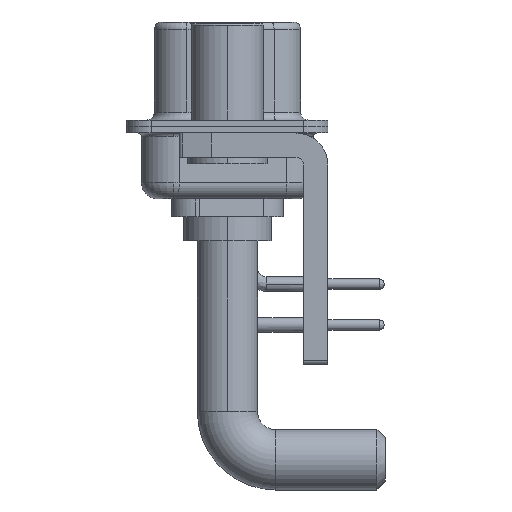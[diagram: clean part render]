
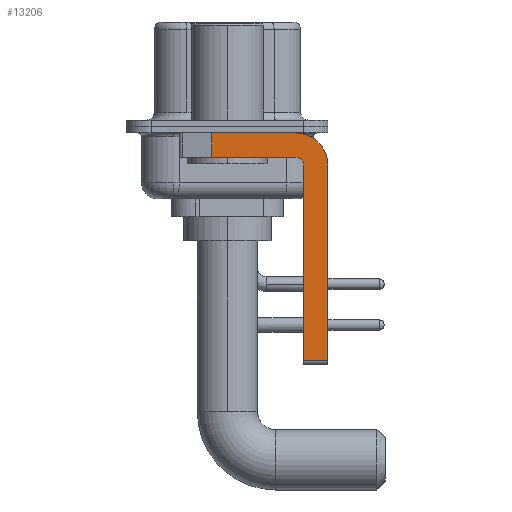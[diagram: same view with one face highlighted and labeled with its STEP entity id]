
A CAD part, left-side view. The second image highlights one B-rep face of the part: STEP entity #13206.
In plain terms, the highlighted planar face has unit normal (-1, 0, 0).
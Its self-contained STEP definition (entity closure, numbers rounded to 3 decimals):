
#13 = ORIENTED_EDGE ( 'NONE', *, *, #18868, .T. ) ;
#313 = ORIENTED_EDGE ( 'NONE', *, *, #8217, .F. ) ;
#1547 = LINE ( 'NONE', #5778, #13247 ) ;
#1688 = VERTEX_POINT ( 'NONE', #19954 ) ;
#1714 = CARTESIAN_POINT ( 'NONE',  ( -2.9, -4.25, -2.4 ) ) ;
#1807 = AXIS2_PLACEMENT_3D ( 'NONE', #6169, #8895, #23213 ) ;
#2792 = EDGE_CURVE ( 'NONE', #22148, #3441, #10200, .T. ) ;
#3090 = ORIENTED_EDGE ( 'NONE', *, *, #12988, .T. ) ;
#3268 = CARTESIAN_POINT ( 'NONE',  ( -2.9, 0.978, -0.4 ) ) ;
#3317 = DIRECTION ( 'NONE',  ( 0., -1., 0. ) ) ;
#3441 = VERTEX_POINT ( 'NONE', #26065 ) ;
#3748 = CARTESIAN_POINT ( 'NONE',  ( -2.9, -4.25, -1.9 ) ) ;
#3822 = CARTESIAN_POINT ( 'NONE',  ( -2.9, -4.25, -1.9 ) ) ;
#3893 = CARTESIAN_POINT ( 'NONE',  ( -2.9, -4.25, -0.4 ) ) ;
#4462 = VERTEX_POINT ( 'NONE', #10042 ) ;
#5024 = AXIS2_PLACEMENT_3D ( 'NONE', #24545, #5852, #7634 ) ;
#5320 = VECTOR ( 'NONE', #10472, 1000. ) ;
#5778 = CARTESIAN_POINT ( 'NONE',  ( -2.9, -4.25, -14.55 ) ) ;
#5852 = DIRECTION ( 'NONE',  ( -1., 0., 0. ) ) ;
#6034 = CARTESIAN_POINT ( 'NONE',  ( -2.9, -6.25, -2.4 ) ) ;
#6169 = CARTESIAN_POINT ( 'NONE',  ( -2.9, -4.25, -2.4 ) ) ;
#6187 = DIRECTION ( 'NONE',  ( 0., 0., -1. ) ) ;
#6374 = VECTOR ( 'NONE', #11959, 1000. ) ;
#6579 = LINE ( 'NONE', #23232, #15756 ) ;
#6833 = EDGE_CURVE ( 'NONE', #8709, #26379, #17943, .T. ) ;
#7211 = VECTOR ( 'NONE', #3317, 1000. ) ;
#7634 = DIRECTION ( 'NONE',  ( 0., 0., 1. ) ) ;
#8217 = EDGE_CURVE ( 'NONE', #25365, #16747, #22420, .T. ) ;
#8627 = PLANE ( 'NONE',  #1807 ) ;
#8709 = VERTEX_POINT ( 'NONE', #3822 ) ;
#8895 = DIRECTION ( 'NONE',  ( 1., 0., 0. ) ) ;
#10042 = CARTESIAN_POINT ( 'NONE',  ( -2.9, -4.75, -2.4 ) ) ;
#10200 = LINE ( 'NONE', #26837, #5320 ) ;
#10472 = DIRECTION ( 'NONE',  ( 0., 0., -1. ) ) ;
#11743 = LINE ( 'NONE', #18270, #22120 ) ;
#11871 = DIRECTION ( 'NONE',  ( 0., 0., 1. ) ) ;
#11959 = DIRECTION ( 'NONE',  ( 0., 1., 0. ) ) ;
#12988 = EDGE_CURVE ( 'NONE', #25365, #26379, #6579, .T. ) ;
#13206 = ADVANCED_FACE ( 'NONE', ( #25126 ), #8627, .F. ) ;
#13247 = VECTOR ( 'NONE', #22174, 1000. ) ;
#13322 = EDGE_LOOP ( 'NONE', ( #313, #3090, #19297, #14415, #20911, #13, #19116, #15576 ) ) ;
#13759 = CIRCLE ( 'NONE', #5024, 0.5 ) ;
#14134 = DIRECTION ( 'NONE',  ( 1., 0., 0. ) ) ;
#14415 = ORIENTED_EDGE ( 'NONE', *, *, #20709, .F. ) ;
#15576 = ORIENTED_EDGE ( 'NONE', *, *, #18301, .F. ) ;
#15756 = VECTOR ( 'NONE', #6187, 1000. ) ;
#16747 = VERTEX_POINT ( 'NONE', #3893 ) ;
#17943 = LINE ( 'NONE', #3748, #6374 ) ;
#18270 = CARTESIAN_POINT ( 'NONE',  ( -2.9, -4.75, -14.8 ) ) ;
#18301 = EDGE_CURVE ( 'NONE', #16747, #22148, #18462, .T. ) ;
#18462 = CIRCLE ( 'NONE', #20640, 2. ) ;
#18868 = EDGE_CURVE ( 'NONE', #1688, #3441, #1547, .T. ) ;
#19116 = ORIENTED_EDGE ( 'NONE', *, *, #2792, .F. ) ;
#19297 = ORIENTED_EDGE ( 'NONE', *, *, #6833, .F. ) ;
#19954 = CARTESIAN_POINT ( 'NONE',  ( -2.9, -4.75, -14.55 ) ) ;
#20640 = AXIS2_PLACEMENT_3D ( 'NONE', #1714, #14134, #22456 ) ;
#20709 = EDGE_CURVE ( 'NONE', #4462, #8709, #13759, .T. ) ;
#20911 = ORIENTED_EDGE ( 'NONE', *, *, #26814, .F. ) ;
#22020 = CARTESIAN_POINT ( 'NONE',  ( -2.9, 3., -0.4 ) ) ;
#22120 = VECTOR ( 'NONE', #11871, 1000. ) ;
#22148 = VERTEX_POINT ( 'NONE', #6034 ) ;
#22174 = DIRECTION ( 'NONE',  ( 0., -1., 0. ) ) ;
#22420 = LINE ( 'NONE', #22020, #7211 ) ;
#22456 = DIRECTION ( 'NONE',  ( 0., 0., -1. ) ) ;
#23213 = DIRECTION ( 'NONE',  ( 0., 0., -1. ) ) ;
#23232 = CARTESIAN_POINT ( 'NONE',  ( -2.9, 0.978, -1.9 ) ) ;
#23496 = CARTESIAN_POINT ( 'NONE',  ( -2.9, 0.978, -1.9 ) ) ;
#24545 = CARTESIAN_POINT ( 'NONE',  ( -2.9, -4.25, -2.4 ) ) ;
#25126 = FACE_OUTER_BOUND ( 'NONE', #13322, .T. ) ;
#25365 = VERTEX_POINT ( 'NONE', #3268 ) ;
#26065 = CARTESIAN_POINT ( 'NONE',  ( -2.9, -6.25, -14.55 ) ) ;
#26379 = VERTEX_POINT ( 'NONE', #23496 ) ;
#26814 = EDGE_CURVE ( 'NONE', #1688, #4462, #11743, .T. ) ;
#26837 = CARTESIAN_POINT ( 'NONE',  ( -2.9, -6.25, -2.4 ) ) ;
